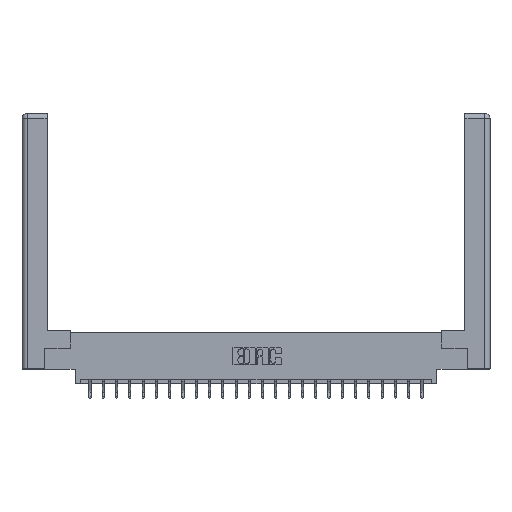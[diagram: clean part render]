
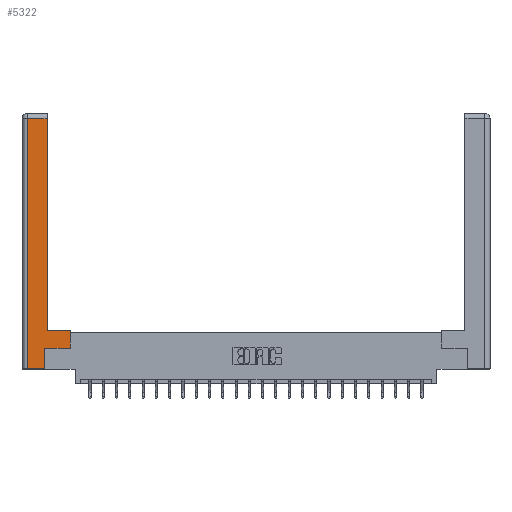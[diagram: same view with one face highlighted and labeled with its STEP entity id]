
A CAD part, top view. The second image highlights one B-rep face of the part: STEP entity #5322.
In plain terms, the highlighted planar face has unit normal (0, 0, 1).
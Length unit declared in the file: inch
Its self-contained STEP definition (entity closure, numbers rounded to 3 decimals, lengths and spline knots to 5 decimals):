
#70 = CARTESIAN_POINT ( 'NONE',  ( 0.565, 0.245, 0. ) ) ;
#122 = EDGE_CURVE ( 'NONE', #8646, #21856, #24342, .T. ) ;
#331 = CARTESIAN_POINT ( 'NONE',  ( 0.565, 0.45, 0. ) ) ;
#2093 = ORIENTED_EDGE ( 'NONE', *, *, #16225, .T. ) ;
#2121 = DIRECTION ( 'NONE',  ( 0., 1., 0. ) ) ;
#2355 = DIRECTION ( 'NONE',  ( 1., 0., 0. ) ) ;
#2469 = DIRECTION ( 'NONE',  ( 0., 1., 0. ) ) ;
#2525 = LINE ( 'NONE', #16242, #24438 ) ;
#2536 = CARTESIAN_POINT ( 'NONE',  ( 0.0615, 0., 0. ) ) ;
#2627 = CARTESIAN_POINT ( 'NONE',  ( 0.295, 3., 0. ) ) ;
#2983 = PLANE ( 'NONE',  #24627 ) ;
#3313 = ORIENTED_EDGE ( 'NONE', *, *, #10016, .T. ) ;
#3903 = EDGE_CURVE ( 'NONE', #18484, #10383, #4971, .T. ) ;
#4917 = VECTOR ( 'NONE', #22288, 39.37008 ) ;
#4932 = ORIENTED_EDGE ( 'NONE', *, *, #3903, .T. ) ;
#4971 = LINE ( 'NONE', #23537, #10182 ) ;
#5033 = CARTESIAN_POINT ( 'NONE',  ( 0., 0., 0. ) ) ;
#5294 = LINE ( 'NONE', #331, #6198 ) ;
#5322 = ADVANCED_FACE ( 'NONE', ( #24691 ), #2983, .F. ) ;
#5999 = VERTEX_POINT ( 'NONE', #70 ) ;
#6198 = VECTOR ( 'NONE', #14571, 39.37008 ) ;
#7094 = CARTESIAN_POINT ( 'NONE',  ( 0.295, 0.45, 0. ) ) ;
#8093 = CARTESIAN_POINT ( 'NONE',  ( 0.0615, 2.94, 0. ) ) ;
#8464 = EDGE_CURVE ( 'NONE', #21856, #9833, #10118, .T. ) ;
#8646 = VERTEX_POINT ( 'NONE', #7094 ) ;
#9157 = CARTESIAN_POINT ( 'NONE',  ( 0.265, 0., 0. ) ) ;
#9833 = VERTEX_POINT ( 'NONE', #8093 ) ;
#10016 = EDGE_CURVE ( 'NONE', #13647, #18484, #13115, .T. ) ;
#10118 = LINE ( 'NONE', #10177, #4917 ) ;
#10177 = CARTESIAN_POINT ( 'NONE',  ( 0.0615, 2.94, 0. ) ) ;
#10182 = VECTOR ( 'NONE', #2121, 39.37008 ) ;
#10321 = ORIENTED_EDGE ( 'NONE', *, *, #18616, .T. ) ;
#10383 = VERTEX_POINT ( 'NONE', #16789 ) ;
#10542 = CARTESIAN_POINT ( 'NONE',  ( 0.295, 2.94, 0. ) ) ;
#10597 = DIRECTION ( 'NONE',  ( -1., 0., 0. ) ) ;
#11794 = DIRECTION ( 'NONE',  ( -1., 0., 0. ) ) ;
#12836 = LINE ( 'NONE', #25242, #16154 ) ;
#12839 = DIRECTION ( 'NONE',  ( 0., 0., -1. ) ) ;
#13115 = LINE ( 'NONE', #9157, #20362 ) ;
#13647 = VERTEX_POINT ( 'NONE', #2536 ) ;
#14571 = DIRECTION ( 'NONE',  ( 0., 1., 0. ) ) ;
#15362 = EDGE_LOOP ( 'NONE', ( #15735, #23944, #10321, #3313, #4932, #2093, #16544, #17506 ) ) ;
#15735 = ORIENTED_EDGE ( 'NONE', *, *, #122, .T. ) ;
#15818 = LINE ( 'NONE', #19842, #24902 ) ;
#16118 = EDGE_CURVE ( 'NONE', #5999, #20489, #5294, .T. ) ;
#16154 = VECTOR ( 'NONE', #17365, 39.37008 ) ;
#16225 = EDGE_CURVE ( 'NONE', #10383, #5999, #2525, .T. ) ;
#16242 = CARTESIAN_POINT ( 'NONE',  ( 0.565, 0.245, 0. ) ) ;
#16544 = ORIENTED_EDGE ( 'NONE', *, *, #16118, .T. ) ;
#16789 = CARTESIAN_POINT ( 'NONE',  ( 0.265, 0.245, 0. ) ) ;
#17365 = DIRECTION ( 'NONE',  ( 0., -1., 0. ) ) ;
#17506 = ORIENTED_EDGE ( 'NONE', *, *, #21193, .T. ) ;
#18484 = VERTEX_POINT ( 'NONE', #24905 ) ;
#18616 = EDGE_CURVE ( 'NONE', #9833, #13647, #12836, .T. ) ;
#19433 = CARTESIAN_POINT ( 'NONE',  ( 0.565, 0.45, 0. ) ) ;
#19842 = CARTESIAN_POINT ( 'NONE',  ( 0.295, 0.45, 0. ) ) ;
#20362 = VECTOR ( 'NONE', #24960, 39.37008 ) ;
#20489 = VERTEX_POINT ( 'NONE', #19433 ) ;
#21193 = EDGE_CURVE ( 'NONE', #20489, #8646, #15818, .T. ) ;
#21856 = VERTEX_POINT ( 'NONE', #10542 ) ;
#22288 = DIRECTION ( 'NONE',  ( -1., 0., 0. ) ) ;
#23537 = CARTESIAN_POINT ( 'NONE',  ( 0.265, 0.245, 0. ) ) ;
#23944 = ORIENTED_EDGE ( 'NONE', *, *, #8464, .T. ) ;
#24020 = VECTOR ( 'NONE', #2469, 39.37008 ) ;
#24342 = LINE ( 'NONE', #2627, #24020 ) ;
#24438 = VECTOR ( 'NONE', #2355, 39.37008 ) ;
#24627 = AXIS2_PLACEMENT_3D ( 'NONE', #5033, #12839, #10597 ) ;
#24691 = FACE_OUTER_BOUND ( 'NONE', #15362, .T. ) ;
#24902 = VECTOR ( 'NONE', #11794, 39.37008 ) ;
#24905 = CARTESIAN_POINT ( 'NONE',  ( 0.265, 0., 0. ) ) ;
#24960 = DIRECTION ( 'NONE',  ( 1., 0., 0. ) ) ;
#25242 = CARTESIAN_POINT ( 'NONE',  ( 0.0615, 0., 0. ) ) ;
